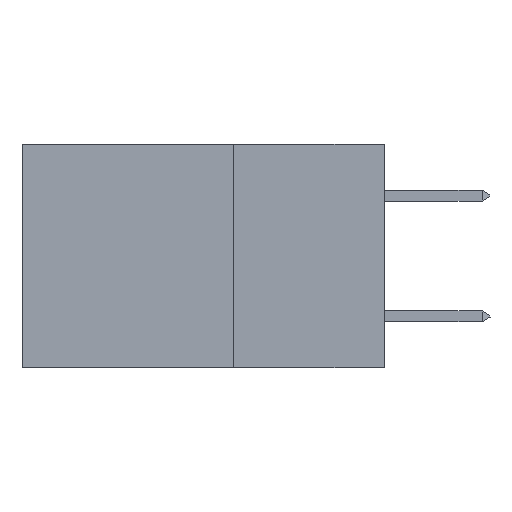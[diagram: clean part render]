
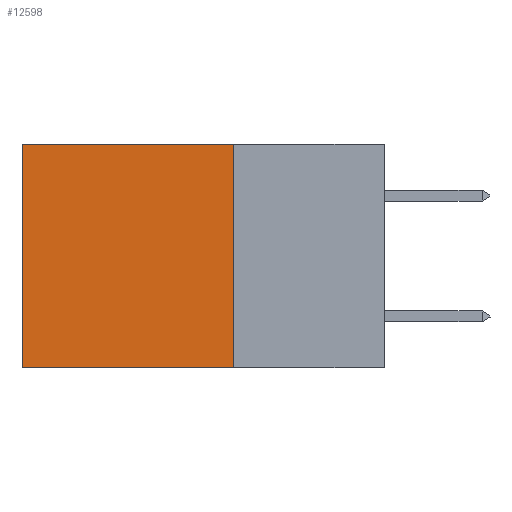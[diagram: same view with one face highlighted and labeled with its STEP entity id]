
A CAD part, left-side view. The second image highlights one B-rep face of the part: STEP entity #12598.
In plain terms, the highlighted planar face has unit normal (-1, 0, 0).
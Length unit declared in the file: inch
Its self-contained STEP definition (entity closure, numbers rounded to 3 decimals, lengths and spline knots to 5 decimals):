
#926 = DIRECTION ( 'NONE',  ( 1., 0., 0. ) ) ;
#1196 = EDGE_CURVE ( 'NONE', #16998, #12435, #10203, .T. ) ;
#1272 = DIRECTION ( 'NONE',  ( 0., 1., 0. ) ) ;
#1278 = ORIENTED_EDGE ( 'NONE', *, *, #1196, .F. ) ;
#1658 = CARTESIAN_POINT ( 'NONE',  ( 0.2875, 0.6, 0. ) ) ;
#1985 = VERTEX_POINT ( 'NONE', #1658 ) ;
#2326 = FACE_OUTER_BOUND ( 'NONE', #12828, .T. ) ;
#2415 = VECTOR ( 'NONE', #12049, 39.37008 ) ;
#2555 = EDGE_CURVE ( 'NONE', #4319, #1985, #16711, .T. ) ;
#3021 = ORIENTED_EDGE ( 'NONE', *, *, #2555, .T. ) ;
#3251 = CARTESIAN_POINT ( 'NONE',  ( 0.2875, 0.25, -0.37 ) ) ;
#4319 = VERTEX_POINT ( 'NONE', #5645 ) ;
#4479 = VECTOR ( 'NONE', #4926, 39.37008 ) ;
#4926 = DIRECTION ( 'NONE',  ( 0., 0., -1. ) ) ;
#5606 = EDGE_CURVE ( 'NONE', #4319, #16998, #9181, .T. ) ;
#5645 = CARTESIAN_POINT ( 'NONE',  ( 0.2875, 0.25, 0. ) ) ;
#6793 = EDGE_CURVE ( 'NONE', #1985, #12435, #11660, .T. ) ;
#7244 = DIRECTION ( 'NONE',  ( 0., 1., 0. ) ) ;
#7299 = CARTESIAN_POINT ( 'NONE',  ( 0.2875, 0.6, 0. ) ) ;
#7447 = VECTOR ( 'NONE', #7244, 39.37008 ) ;
#7971 = CARTESIAN_POINT ( 'NONE',  ( 0.2875, 0.25, 0. ) ) ;
#8028 = VECTOR ( 'NONE', #1272, 39.37008 ) ;
#9181 = LINE ( 'NONE', #7971, #2415 ) ;
#10203 = LINE ( 'NONE', #3251, #7447 ) ;
#11196 = AXIS2_PLACEMENT_3D ( 'NONE', #15720, #926, #15597 ) ;
#11571 = PLANE ( 'NONE',  #11196 ) ;
#11660 = LINE ( 'NONE', #7299, #4479 ) ;
#12049 = DIRECTION ( 'NONE',  ( 0., 0., -1. ) ) ;
#12435 = VERTEX_POINT ( 'NONE', #17330 ) ;
#12598 = ADVANCED_FACE ( 'NONE', ( #2326 ), #11571, .F. ) ;
#12828 = EDGE_LOOP ( 'NONE', ( #16050, #1278, #15506, #3021 ) ) ;
#13622 = CARTESIAN_POINT ( 'NONE',  ( 0.2875, 0.25, 0. ) ) ;
#15506 = ORIENTED_EDGE ( 'NONE', *, *, #5606, .F. ) ;
#15597 = DIRECTION ( 'NONE',  ( 0., 0., -1. ) ) ;
#15720 = CARTESIAN_POINT ( 'NONE',  ( 0.2875, 0.25, 0. ) ) ;
#15886 = CARTESIAN_POINT ( 'NONE',  ( 0.2875, 0.25, -0.37 ) ) ;
#16050 = ORIENTED_EDGE ( 'NONE', *, *, #6793, .T. ) ;
#16711 = LINE ( 'NONE', #13622, #8028 ) ;
#16998 = VERTEX_POINT ( 'NONE', #15886 ) ;
#17330 = CARTESIAN_POINT ( 'NONE',  ( 0.2875, 0.6, -0.37 ) ) ;
